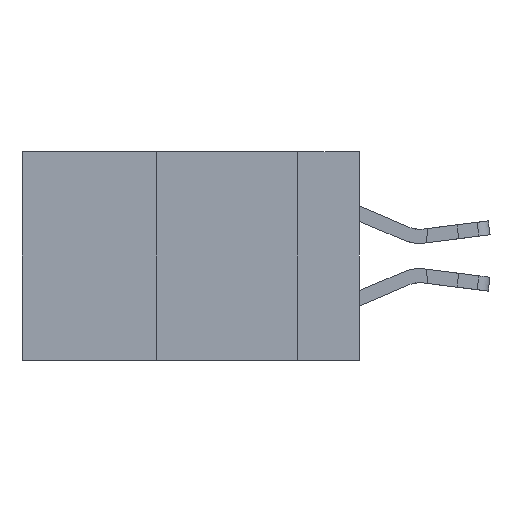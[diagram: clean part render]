
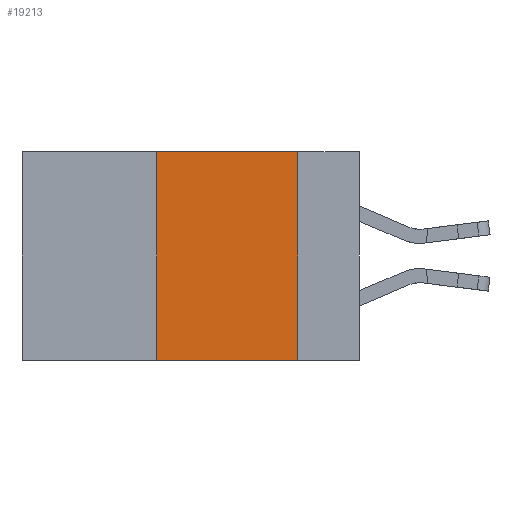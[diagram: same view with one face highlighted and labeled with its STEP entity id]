
A CAD part, left-side view. The second image highlights one B-rep face of the part: STEP entity #19213.
In plain terms, the highlighted planar face has unit normal (-1, 0, 0).
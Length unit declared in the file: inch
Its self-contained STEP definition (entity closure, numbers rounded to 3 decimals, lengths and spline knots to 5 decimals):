
#1037 = CARTESIAN_POINT ( 'NONE',  ( 0., 0.36, -0.37 ) ) ;
#1416 = LINE ( 'NONE', #11489, #17173 ) ;
#1609 = VECTOR ( 'NONE', #24143, 39.37008 ) ;
#2171 = DIRECTION ( 'NONE',  ( 0., -1., 0. ) ) ;
#2355 = CARTESIAN_POINT ( 'NONE',  ( 0., 0.6, 0. ) ) ;
#2653 = VERTEX_POINT ( 'NONE', #13633 ) ;
#2825 = CARTESIAN_POINT ( 'NONE',  ( 0., 0.36, 0. ) ) ;
#4686 = LINE ( 'NONE', #2355, #1609 ) ;
#5508 = FACE_OUTER_BOUND ( 'NONE', #7094, .T. ) ;
#5613 = ORIENTED_EDGE ( 'NONE', *, *, #8990, .F. ) ;
#6477 = DIRECTION ( 'NONE',  ( 1., 0., 0. ) ) ;
#6775 = VERTEX_POINT ( 'NONE', #1037 ) ;
#7094 = EDGE_LOOP ( 'NONE', ( #17458, #5613, #14864, #11348 ) ) ;
#7495 = CARTESIAN_POINT ( 'NONE',  ( 0., 0.11, 0. ) ) ;
#7617 = DIRECTION ( 'NONE',  ( 0., 0., -1. ) ) ;
#8188 = VECTOR ( 'NONE', #16711, 39.37008 ) ;
#8990 = EDGE_CURVE ( 'NONE', #2653, #11758, #4686, .T. ) ;
#10166 = CARTESIAN_POINT ( 'NONE',  ( 0., 0.6, -0.37 ) ) ;
#10791 = VERTEX_POINT ( 'NONE', #19056 ) ;
#11348 = ORIENTED_EDGE ( 'NONE', *, *, #11501, .T. ) ;
#11489 = CARTESIAN_POINT ( 'NONE',  ( 0., 0.11, 0. ) ) ;
#11501 = EDGE_CURVE ( 'NONE', #6775, #10791, #23067, .T. ) ;
#11758 = VERTEX_POINT ( 'NONE', #7495 ) ;
#12252 = CARTESIAN_POINT ( 'NONE',  ( 0., 0.6, 0. ) ) ;
#13020 = EDGE_CURVE ( 'NONE', #6775, #2653, #13439, .T. ) ;
#13439 = LINE ( 'NONE', #2825, #8188 ) ;
#13633 = CARTESIAN_POINT ( 'NONE',  ( 0., 0.36, 0. ) ) ;
#14864 = ORIENTED_EDGE ( 'NONE', *, *, #13020, .F. ) ;
#16711 = DIRECTION ( 'NONE',  ( 0., 0., 1. ) ) ;
#17173 = VECTOR ( 'NONE', #7617, 39.37008 ) ;
#17458 = ORIENTED_EDGE ( 'NONE', *, *, #23096, .F. ) ;
#18208 = PLANE ( 'NONE',  #22416 ) ;
#19056 = CARTESIAN_POINT ( 'NONE',  ( 0., 0.11, -0.37 ) ) ;
#19213 = ADVANCED_FACE ( 'NONE', ( #5508 ), #18208, .F. ) ;
#21200 = VECTOR ( 'NONE', #2171, 39.37008 ) ;
#22069 = DIRECTION ( 'NONE',  ( 0., 0., -1. ) ) ;
#22416 = AXIS2_PLACEMENT_3D ( 'NONE', #12252, #6477, #22069 ) ;
#23067 = LINE ( 'NONE', #10166, #21200 ) ;
#23096 = EDGE_CURVE ( 'NONE', #11758, #10791, #1416, .T. ) ;
#24143 = DIRECTION ( 'NONE',  ( 0., -1., 0. ) ) ;
